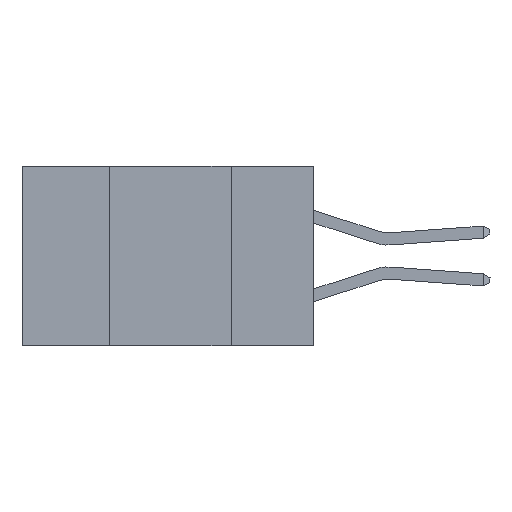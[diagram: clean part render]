
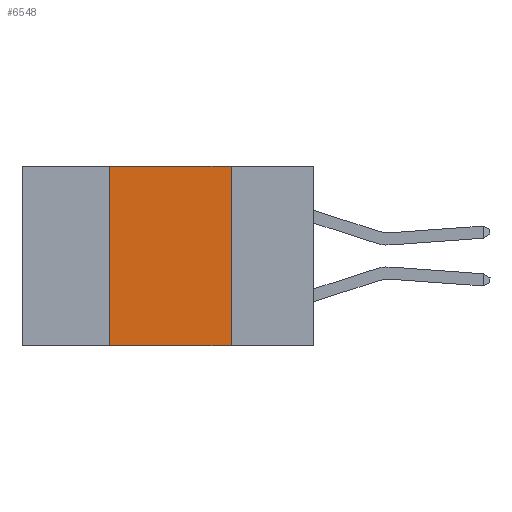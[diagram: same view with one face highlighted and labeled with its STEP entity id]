
A CAD part, left-side view. The second image highlights one B-rep face of the part: STEP entity #6548.
In plain terms, the highlighted planar face has unit normal (-1, 0, 0).
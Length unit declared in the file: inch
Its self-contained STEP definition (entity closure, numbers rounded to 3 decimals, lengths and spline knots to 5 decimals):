
#365 = PLANE ( 'NONE',  #15975 ) ;
#628 = VERTEX_POINT ( 'NONE', #10454 ) ;
#1135 = ORIENTED_EDGE ( 'NONE', *, *, #5662, .F. ) ;
#1522 = CARTESIAN_POINT ( 'NONE',  ( 0., 0.6, -0.37 ) ) ;
#2223 = VERTEX_POINT ( 'NONE', #18145 ) ;
#2328 = CARTESIAN_POINT ( 'NONE',  ( 0., 0.6, 0. ) ) ;
#2600 = ORIENTED_EDGE ( 'NONE', *, *, #3580, .F. ) ;
#2706 = VECTOR ( 'NONE', #19588, 39.37008 ) ;
#3439 = EDGE_LOOP ( 'NONE', ( #1135, #13678, #2600, #3750 ) ) ;
#3580 = EDGE_CURVE ( 'NONE', #12679, #8018, #19360, .T. ) ;
#3629 = CARTESIAN_POINT ( 'NONE',  ( 0., 0.6, 0. ) ) ;
#3750 = ORIENTED_EDGE ( 'NONE', *, *, #15436, .T. ) ;
#4050 = LINE ( 'NONE', #1522, #20160 ) ;
#4458 = CARTESIAN_POINT ( 'NONE',  ( 0., 0.42, 0. ) ) ;
#4641 = DIRECTION ( 'NONE',  ( 0., 0., 1. ) ) ;
#4966 = EDGE_CURVE ( 'NONE', #8018, #2223, #7100, .T. ) ;
#5662 = EDGE_CURVE ( 'NONE', #2223, #628, #18057, .T. ) ;
#6548 = ADVANCED_FACE ( 'NONE', ( #7062 ), #365, .F. ) ;
#7062 = FACE_OUTER_BOUND ( 'NONE', #3439, .T. ) ;
#7100 = LINE ( 'NONE', #2328, #2706 ) ;
#8018 = VERTEX_POINT ( 'NONE', #11530 ) ;
#8155 = DIRECTION ( 'NONE',  ( 0., 0., -1. ) ) ;
#10454 = CARTESIAN_POINT ( 'NONE',  ( 0., 0.17, -0.37 ) ) ;
#11241 = VECTOR ( 'NONE', #8155, 39.37008 ) ;
#11530 = CARTESIAN_POINT ( 'NONE',  ( 0., 0.42, 0. ) ) ;
#12542 = VECTOR ( 'NONE', #4641, 39.37008 ) ;
#12679 = VERTEX_POINT ( 'NONE', #15870 ) ;
#13637 = DIRECTION ( 'NONE',  ( 1., 0., 0. ) ) ;
#13678 = ORIENTED_EDGE ( 'NONE', *, *, #4966, .F. ) ;
#14371 = CARTESIAN_POINT ( 'NONE',  ( 0., 0.17, 0. ) ) ;
#15436 = EDGE_CURVE ( 'NONE', #12679, #628, #4050, .T. ) ;
#15870 = CARTESIAN_POINT ( 'NONE',  ( 0., 0.42, -0.37 ) ) ;
#15975 = AXIS2_PLACEMENT_3D ( 'NONE', #3629, #13637, #16781 ) ;
#16781 = DIRECTION ( 'NONE',  ( 0., 0., -1. ) ) ;
#17137 = DIRECTION ( 'NONE',  ( 0., -1., 0. ) ) ;
#18057 = LINE ( 'NONE', #14371, #11241 ) ;
#18145 = CARTESIAN_POINT ( 'NONE',  ( 0., 0.17, 0. ) ) ;
#19360 = LINE ( 'NONE', #4458, #12542 ) ;
#19588 = DIRECTION ( 'NONE',  ( 0., -1., 0. ) ) ;
#20160 = VECTOR ( 'NONE', #17137, 39.37008 ) ;
